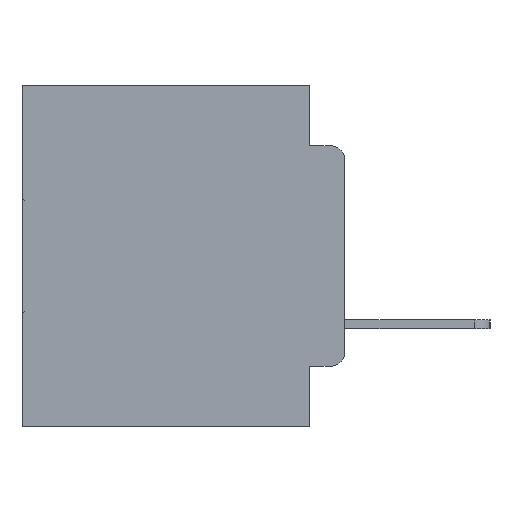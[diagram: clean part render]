
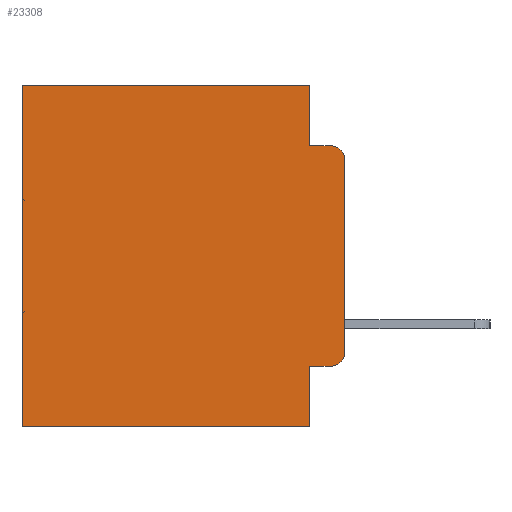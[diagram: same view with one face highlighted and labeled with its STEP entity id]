
A CAD part, left-side view. The second image highlights one B-rep face of the part: STEP entity #23308.
In plain terms, the highlighted planar face has unit normal (-1, 0, 0).
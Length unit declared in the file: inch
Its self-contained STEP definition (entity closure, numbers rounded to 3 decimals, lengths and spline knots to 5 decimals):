
#42 = LINE ( 'NONE', #16532, #29713 ) ;
#428 = ORIENTED_EDGE ( 'NONE', *, *, #16030, .T. ) ;
#885 = VECTOR ( 'NONE', #29651, 39.37008 ) ;
#1967 = PLANE ( 'NONE',  #27192 ) ;
#2775 = EDGE_LOOP ( 'NONE', ( #6258, #428, #13523, #24031, #18243, #27712, #28835, #12776, #24463, #5405 ) ) ;
#3248 = LINE ( 'NONE', #6320, #10290 ) ;
#4025 = DIRECTION ( 'NONE',  ( 0., 0., -1. ) ) ;
#5233 = LINE ( 'NONE', #20521, #30097 ) ;
#5405 = ORIENTED_EDGE ( 'NONE', *, *, #23279, .T. ) ;
#5618 = CARTESIAN_POINT ( 'NONE',  ( 0.298, 0., -0.5 ) ) ;
#5750 = LINE ( 'NONE', #26487, #29876 ) ;
#6051 = CARTESIAN_POINT ( 'NONE',  ( 0.298, 0.02, -0.0885 ) ) ;
#6056 = CARTESIAN_POINT ( 'NONE',  ( 0.298, 0.02, -0.1085 ) ) ;
#6069 = VERTEX_POINT ( 'NONE', #20152 ) ;
#6258 = ORIENTED_EDGE ( 'NONE', *, *, #8782, .F. ) ;
#6310 = EDGE_CURVE ( 'NONE', #8501, #8920, #3248, .T. ) ;
#6320 = CARTESIAN_POINT ( 'NONE',  ( 0.298, 0.051, 0. ) ) ;
#6696 = CARTESIAN_POINT ( 'NONE',  ( 0.298, 0., -0.3915 ) ) ;
#7062 = DIRECTION ( 'NONE',  ( 0., 0., -1. ) ) ;
#7342 = VECTOR ( 'NONE', #11982, 39.37008 ) ;
#8448 = DIRECTION ( 'NONE',  ( 0., 0., -1. ) ) ;
#8501 = VERTEX_POINT ( 'NONE', #10061 ) ;
#8782 = EDGE_CURVE ( 'NONE', #11065, #24695, #5233, .T. ) ;
#8920 = VERTEX_POINT ( 'NONE', #18668 ) ;
#9085 = CARTESIAN_POINT ( 'NONE',  ( 0.298, 0., 0. ) ) ;
#9512 = DIRECTION ( 'NONE',  ( 0., 0., -1. ) ) ;
#9682 = EDGE_CURVE ( 'NONE', #14597, #25173, #25380, .T. ) ;
#9813 = CARTESIAN_POINT ( 'NONE',  ( 0.298, 0.051, -0.0885 ) ) ;
#10061 = CARTESIAN_POINT ( 'NONE',  ( 0.298, 0.051, -0.4115 ) ) ;
#10290 = VECTOR ( 'NONE', #7062, 39.37008 ) ;
#10298 = CIRCLE ( 'NONE', #17363, 0.02 ) ;
#10490 = CARTESIAN_POINT ( 'NONE',  ( 0.298, 0., -0.1085 ) ) ;
#11065 = VERTEX_POINT ( 'NONE', #10490 ) ;
#11428 = DIRECTION ( 'NONE',  ( -1., 0., 0. ) ) ;
#11538 = DIRECTION ( 'NONE',  ( 1., 0., 0. ) ) ;
#11563 = VECTOR ( 'NONE', #26164, 39.37008 ) ;
#11617 = EDGE_CURVE ( 'NONE', #19181, #19148, #5750, .T. ) ;
#11982 = DIRECTION ( 'NONE',  ( 0., -1., 0. ) ) ;
#12575 = DIRECTION ( 'NONE',  ( 0., 1., 0. ) ) ;
#12776 = ORIENTED_EDGE ( 'NONE', *, *, #6310, .F. ) ;
#13457 = CARTESIAN_POINT ( 'NONE',  ( 0.298, 0.051, 0. ) ) ;
#13523 = ORIENTED_EDGE ( 'NONE', *, *, #9682, .F. ) ;
#14308 = EDGE_CURVE ( 'NONE', #19148, #19494, #42, .T. ) ;
#14597 = VERTEX_POINT ( 'NONE', #25034 ) ;
#16024 = CARTESIAN_POINT ( 'NONE',  ( 0.298, 0.051, 0. ) ) ;
#16030 = EDGE_CURVE ( 'NONE', #11065, #25173, #10298, .T. ) ;
#16532 = CARTESIAN_POINT ( 'NONE',  ( 0.298, 0.473, 0. ) ) ;
#17363 = AXIS2_PLACEMENT_3D ( 'NONE', #6056, #22505, #8448 ) ;
#18243 = ORIENTED_EDGE ( 'NONE', *, *, #11617, .T. ) ;
#18246 = CARTESIAN_POINT ( 'NONE',  ( 0.298, 0.473, 0. ) ) ;
#18668 = CARTESIAN_POINT ( 'NONE',  ( 0.298, 0.051, -0.5 ) ) ;
#19148 = VERTEX_POINT ( 'NONE', #18246 ) ;
#19181 = VERTEX_POINT ( 'NONE', #16024 ) ;
#19494 = VERTEX_POINT ( 'NONE', #22124 ) ;
#20152 = CARTESIAN_POINT ( 'NONE',  ( 0.298, 0.02, -0.4115 ) ) ;
#20440 = LINE ( 'NONE', #13457, #885 ) ;
#20521 = CARTESIAN_POINT ( 'NONE',  ( 0.298, 0., 0. ) ) ;
#20983 = AXIS2_PLACEMENT_3D ( 'NONE', #25351, #11428, #27691 ) ;
#22091 = DIRECTION ( 'NONE',  ( 0., 1., 0. ) ) ;
#22097 = EDGE_CURVE ( 'NONE', #19181, #14597, #20440, .T. ) ;
#22124 = CARTESIAN_POINT ( 'NONE',  ( 0.298, 0.473, -0.5 ) ) ;
#22505 = DIRECTION ( 'NONE',  ( -1., 0., 0. ) ) ;
#23279 = EDGE_CURVE ( 'NONE', #6069, #24695, #26820, .T. ) ;
#23308 = ADVANCED_FACE ( 'NONE', ( #26091 ), #1967, .F. ) ;
#24031 = ORIENTED_EDGE ( 'NONE', *, *, #22097, .F. ) ;
#24186 = EDGE_CURVE ( 'NONE', #8501, #6069, #26039, .T. ) ;
#24463 = ORIENTED_EDGE ( 'NONE', *, *, #24186, .T. ) ;
#24695 = VERTEX_POINT ( 'NONE', #6696 ) ;
#25034 = CARTESIAN_POINT ( 'NONE',  ( 0.298, 0.051, -0.0885 ) ) ;
#25173 = VERTEX_POINT ( 'NONE', #6051 ) ;
#25351 = CARTESIAN_POINT ( 'NONE',  ( 0.298, 0.02, -0.3915 ) ) ;
#25380 = LINE ( 'NONE', #9813, #11563 ) ;
#25892 = CARTESIAN_POINT ( 'NONE',  ( 0.298, 0.051, -0.4115 ) ) ;
#26039 = LINE ( 'NONE', #25892, #7342 ) ;
#26091 = FACE_OUTER_BOUND ( 'NONE', #2775, .T. ) ;
#26164 = DIRECTION ( 'NONE',  ( 0., -1., 0. ) ) ;
#26487 = CARTESIAN_POINT ( 'NONE',  ( 0.298, 0., 0. ) ) ;
#26820 = CIRCLE ( 'NONE', #20983, 0.02 ) ;
#27192 = AXIS2_PLACEMENT_3D ( 'NONE', #9085, #11538, #27785 ) ;
#27691 = DIRECTION ( 'NONE',  ( 0., 0., -1. ) ) ;
#27712 = ORIENTED_EDGE ( 'NONE', *, *, #14308, .T. ) ;
#27785 = DIRECTION ( 'NONE',  ( 0., 0., -1. ) ) ;
#28835 = ORIENTED_EDGE ( 'NONE', *, *, #29728, .F. ) ;
#29207 = LINE ( 'NONE', #5618, #29914 ) ;
#29651 = DIRECTION ( 'NONE',  ( 0., 0., -1. ) ) ;
#29713 = VECTOR ( 'NONE', #9512, 39.37008 ) ;
#29728 = EDGE_CURVE ( 'NONE', #8920, #19494, #29207, .T. ) ;
#29876 = VECTOR ( 'NONE', #12575, 39.37008 ) ;
#29914 = VECTOR ( 'NONE', #22091, 39.37008 ) ;
#30097 = VECTOR ( 'NONE', #4025, 39.37008 ) ;
